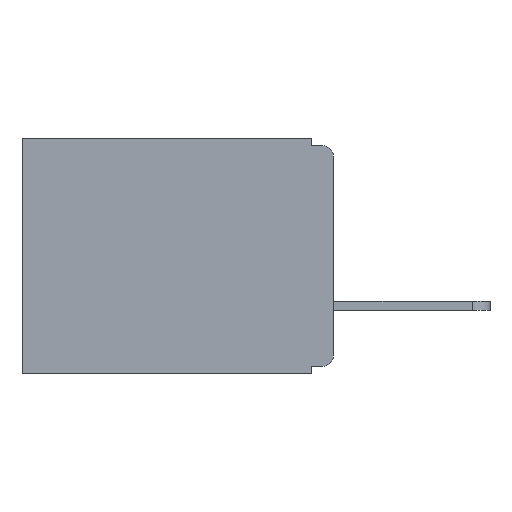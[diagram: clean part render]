
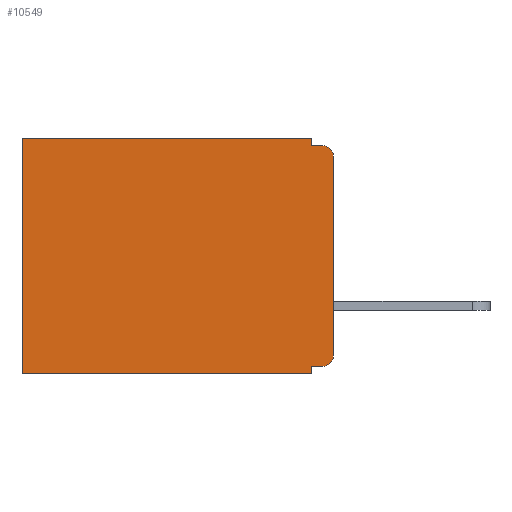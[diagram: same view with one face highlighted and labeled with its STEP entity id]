
A CAD part, left-side view. The second image highlights one B-rep face of the part: STEP entity #10549.
In plain terms, the highlighted planar face has unit normal (-1, 0, 0).
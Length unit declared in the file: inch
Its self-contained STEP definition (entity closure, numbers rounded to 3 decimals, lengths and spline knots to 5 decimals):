
#20 = DIRECTION ( 'NONE',  ( 1., 0., 0. ) ) ;
#276 = ORIENTED_EDGE ( 'NONE', *, *, #10894, .F. ) ;
#685 = CARTESIAN_POINT ( 'NONE',  ( 0.3, 0.015, -0.32 ) ) ;
#754 = CARTESIAN_POINT ( 'NONE',  ( 0.3, 0., -0.33 ) ) ;
#801 = DIRECTION ( 'NONE',  ( 0., 0., -1. ) ) ;
#960 = EDGE_CURVE ( 'NONE', #3314, #5872, #13385, .T. ) ;
#1061 = EDGE_CURVE ( 'NONE', #3314, #11477, #1153, .T. ) ;
#1089 = CARTESIAN_POINT ( 'NONE',  ( 0.3, 0.031, 0. ) ) ;
#1126 = VECTOR ( 'NONE', #4958, 39.37008 ) ;
#1153 = LINE ( 'NONE', #1418, #4769 ) ;
#1325 = VECTOR ( 'NONE', #11146, 39.37008 ) ;
#1418 = CARTESIAN_POINT ( 'NONE',  ( 0.3, 0., -0.32 ) ) ;
#1419 = LINE ( 'NONE', #10982, #2569 ) ;
#1606 = CARTESIAN_POINT ( 'NONE',  ( 0.3, 0., 0. ) ) ;
#2569 = VECTOR ( 'NONE', #12000, 39.37008 ) ;
#2647 = CARTESIAN_POINT ( 'NONE',  ( 0.3, 0.437, -0.33 ) ) ;
#2876 = CARTESIAN_POINT ( 'NONE',  ( 0.3, 0., -0.025 ) ) ;
#3141 = CARTESIAN_POINT ( 'NONE',  ( 0.3, 0., -0.305 ) ) ;
#3286 = AXIS2_PLACEMENT_3D ( 'NONE', #12555, #20, #9406 ) ;
#3294 = EDGE_CURVE ( 'NONE', #9293, #5956, #7376, .T. ) ;
#3314 = VERTEX_POINT ( 'NONE', #685 ) ;
#3404 = DIRECTION ( 'NONE',  ( 0., 0., -1. ) ) ;
#3439 = LINE ( 'NONE', #8584, #3937 ) ;
#3807 = FACE_OUTER_BOUND ( 'NONE', #12816, .T. ) ;
#3859 = CARTESIAN_POINT ( 'NONE',  ( 0.3, 0.437, 0. ) ) ;
#3937 = VECTOR ( 'NONE', #6390, 39.37008 ) ;
#4063 = PLANE ( 'NONE',  #3286 ) ;
#4207 = ORIENTED_EDGE ( 'NONE', *, *, #9171, .T. ) ;
#4304 = VERTEX_POINT ( 'NONE', #9169 ) ;
#4512 = ORIENTED_EDGE ( 'NONE', *, *, #3294, .F. ) ;
#4594 = CARTESIAN_POINT ( 'NONE',  ( 0.3, 0.015, -0.025 ) ) ;
#4618 = AXIS2_PLACEMENT_3D ( 'NONE', #5429, #12838, #3404 ) ;
#4769 = VECTOR ( 'NONE', #6715, 39.37008 ) ;
#4958 = DIRECTION ( 'NONE',  ( 0., 0., -1. ) ) ;
#5141 = CARTESIAN_POINT ( 'NONE',  ( 0.3, 0.031, 0. ) ) ;
#5358 = VERTEX_POINT ( 'NONE', #9319 ) ;
#5429 = CARTESIAN_POINT ( 'NONE',  ( 0.3, 0.015, -0.305 ) ) ;
#5650 = DIRECTION ( 'NONE',  ( -1., 0., 0. ) ) ;
#5651 = CARTESIAN_POINT ( 'NONE',  ( 0.3, 0.031, -0.32 ) ) ;
#5701 = CIRCLE ( 'NONE', #11267, 0.015 ) ;
#5845 = VECTOR ( 'NONE', #13425, 39.37008 ) ;
#5872 = VERTEX_POINT ( 'NONE', #3141 ) ;
#5956 = VERTEX_POINT ( 'NONE', #9552 ) ;
#5999 = ORIENTED_EDGE ( 'NONE', *, *, #10673, .T. ) ;
#6390 = DIRECTION ( 'NONE',  ( 0., -1., 0. ) ) ;
#6490 = EDGE_CURVE ( 'NONE', #10124, #4304, #12528, .T. ) ;
#6715 = DIRECTION ( 'NONE',  ( 0., 1., 0. ) ) ;
#7376 = LINE ( 'NONE', #13390, #8194 ) ;
#7938 = LINE ( 'NONE', #2647, #1325 ) ;
#8194 = VECTOR ( 'NONE', #11202, 39.37008 ) ;
#8328 = ORIENTED_EDGE ( 'NONE', *, *, #8435, .F. ) ;
#8435 = EDGE_CURVE ( 'NONE', #11477, #9293, #1419, .T. ) ;
#8496 = EDGE_CURVE ( 'NONE', #10808, #5358, #5701, .T. ) ;
#8584 = CARTESIAN_POINT ( 'NONE',  ( 0.3, 0., -0.01 ) ) ;
#8921 = VECTOR ( 'NONE', #801, 39.37008 ) ;
#9169 = CARTESIAN_POINT ( 'NONE',  ( 0.3, 0.031, -0.01 ) ) ;
#9171 = EDGE_CURVE ( 'NONE', #10124, #9660, #9807, .T. ) ;
#9293 = VERTEX_POINT ( 'NONE', #11786 ) ;
#9305 = ORIENTED_EDGE ( 'NONE', *, *, #8496, .T. ) ;
#9319 = CARTESIAN_POINT ( 'NONE',  ( 0.3, 0.015, -0.01 ) ) ;
#9406 = DIRECTION ( 'NONE',  ( 0., 0., -1. ) ) ;
#9552 = CARTESIAN_POINT ( 'NONE',  ( 0.3, 0.437, -0.33 ) ) ;
#9660 = VERTEX_POINT ( 'NONE', #3859 ) ;
#9807 = LINE ( 'NONE', #1606, #5845 ) ;
#10124 = VERTEX_POINT ( 'NONE', #1089 ) ;
#10549 = ADVANCED_FACE ( 'NONE', ( #3807 ), #4063, .F. ) ;
#10664 = ORIENTED_EDGE ( 'NONE', *, *, #6490, .F. ) ;
#10673 = EDGE_CURVE ( 'NONE', #9660, #5956, #7938, .T. ) ;
#10789 = ORIENTED_EDGE ( 'NONE', *, *, #960, .T. ) ;
#10808 = VERTEX_POINT ( 'NONE', #2876 ) ;
#10894 = EDGE_CURVE ( 'NONE', #10808, #5872, #11743, .T. ) ;
#10982 = CARTESIAN_POINT ( 'NONE',  ( 0.3, 0.031, -0.33 ) ) ;
#11146 = DIRECTION ( 'NONE',  ( 0., 0., -1. ) ) ;
#11202 = DIRECTION ( 'NONE',  ( 0., 1., 0. ) ) ;
#11267 = AXIS2_PLACEMENT_3D ( 'NONE', #4594, #5650, #11936 ) ;
#11477 = VERTEX_POINT ( 'NONE', #5651 ) ;
#11743 = LINE ( 'NONE', #754, #8921 ) ;
#11786 = CARTESIAN_POINT ( 'NONE',  ( 0.3, 0.031, -0.33 ) ) ;
#11936 = DIRECTION ( 'NONE',  ( 0., 0., -1. ) ) ;
#12000 = DIRECTION ( 'NONE',  ( 0., 0., -1. ) ) ;
#12019 = EDGE_CURVE ( 'NONE', #4304, #5358, #3439, .T. ) ;
#12152 = ORIENTED_EDGE ( 'NONE', *, *, #12019, .F. ) ;
#12493 = ORIENTED_EDGE ( 'NONE', *, *, #1061, .F. ) ;
#12528 = LINE ( 'NONE', #5141, #1126 ) ;
#12555 = CARTESIAN_POINT ( 'NONE',  ( 0.3, 0., -0.33 ) ) ;
#12816 = EDGE_LOOP ( 'NONE', ( #276, #9305, #12152, #10664, #4207, #5999, #4512, #8328, #12493, #10789 ) ) ;
#12838 = DIRECTION ( 'NONE',  ( -1., 0., 0. ) ) ;
#13385 = CIRCLE ( 'NONE', #4618, 0.015 ) ;
#13390 = CARTESIAN_POINT ( 'NONE',  ( 0.3, 0., -0.33 ) ) ;
#13425 = DIRECTION ( 'NONE',  ( 0., 1., 0. ) ) ;
